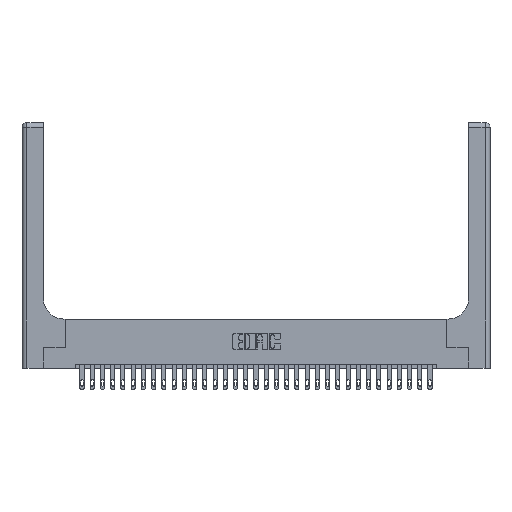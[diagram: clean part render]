
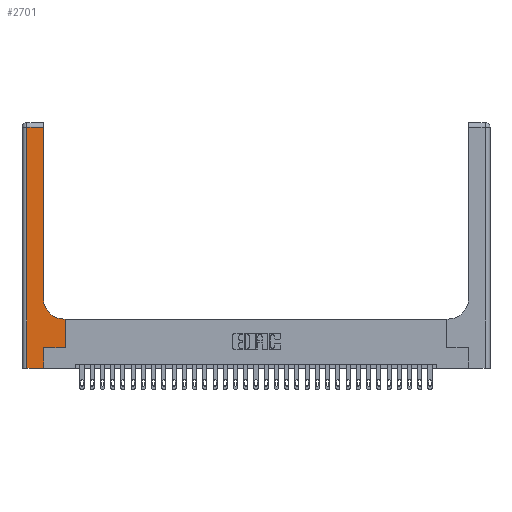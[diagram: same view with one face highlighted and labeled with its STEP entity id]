
A CAD part, top view. The second image highlights one B-rep face of the part: STEP entity #2701.
In plain terms, the highlighted planar face has unit normal (0, 0, 1).
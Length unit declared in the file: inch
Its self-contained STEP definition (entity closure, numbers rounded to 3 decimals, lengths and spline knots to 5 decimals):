
#189 = DIRECTION ( 'NONE',  ( 1., 0., 0. ) ) ;
#437 = LINE ( 'NONE', #23005, #7215 ) ;
#737 = CARTESIAN_POINT ( 'NONE',  ( 0., 0., 0.37 ) ) ;
#1983 = ORIENTED_EDGE ( 'NONE', *, *, #17856, .T. ) ;
#2076 = FACE_OUTER_BOUND ( 'NONE', #5030, .T. ) ;
#2088 = ORIENTED_EDGE ( 'NONE', *, *, #23078, .T. ) ;
#2123 = CARTESIAN_POINT ( 'NONE',  ( 0.265, 0.25, 0.37 ) ) ;
#2350 = CIRCLE ( 'NONE', #26755, 0.25 ) ;
#2701 = ADVANCED_FACE ( 'NONE', ( #2076 ), #20249, .F. ) ;
#3239 = CARTESIAN_POINT ( 'NONE',  ( 0.265, 0., 0.37 ) ) ;
#3316 = DIRECTION ( 'NONE',  ( 0., 0., -1. ) ) ;
#3659 = CARTESIAN_POINT ( 'NONE',  ( 0., 2.94, 0.37 ) ) ;
#3998 = DIRECTION ( 'NONE',  ( 0., 1., 0. ) ) ;
#4167 = VECTOR ( 'NONE', #19620, 39.37008 ) ;
#4446 = DIRECTION ( 'NONE',  ( 0., 0., -1. ) ) ;
#4845 = ORIENTED_EDGE ( 'NONE', *, *, #25050, .T. ) ;
#5030 = EDGE_LOOP ( 'NONE', ( #12765, #10498, #20562, #2088, #4845, #13483, #8958, #1983, #25902 ) ) ;
#5053 = VERTEX_POINT ( 'NONE', #8033 ) ;
#5609 = VECTOR ( 'NONE', #3998, 39.37008 ) ;
#5648 = DIRECTION ( 'NONE',  ( 1., 0., 0. ) ) ;
#6220 = VERTEX_POINT ( 'NONE', #7298 ) ;
#7106 = VECTOR ( 'NONE', #8138, 39.37008 ) ;
#7215 = VECTOR ( 'NONE', #16648, 39.37008 ) ;
#7298 = CARTESIAN_POINT ( 'NONE',  ( 0.528, 0.6, 0.37 ) ) ;
#7432 = CARTESIAN_POINT ( 'NONE',  ( 0.265, 0.25, 0.37 ) ) ;
#8033 = CARTESIAN_POINT ( 'NONE',  ( 0.26, 2.94, 0.37 ) ) ;
#8138 = DIRECTION ( 'NONE',  ( 1., 0., 0. ) ) ;
#8958 = ORIENTED_EDGE ( 'NONE', *, *, #18855, .T. ) ;
#10444 = CARTESIAN_POINT ( 'NONE',  ( 0.51, 0.85, 0.37 ) ) ;
#10498 = ORIENTED_EDGE ( 'NONE', *, *, #15557, .T. ) ;
#10643 = VERTEX_POINT ( 'NONE', #11607 ) ;
#11607 = CARTESIAN_POINT ( 'NONE',  ( 0.06, 2.94, 0.37 ) ) ;
#11711 = VECTOR ( 'NONE', #189, 39.37008 ) ;
#11792 = LINE ( 'NONE', #2123, #11711 ) ;
#12743 = CARTESIAN_POINT ( 'NONE',  ( 0.06, 0., 0.37 ) ) ;
#12765 = ORIENTED_EDGE ( 'NONE', *, *, #24656, .T. ) ;
#13483 = ORIENTED_EDGE ( 'NONE', *, *, #27693, .T. ) ;
#14530 = LINE ( 'NONE', #28483, #4167 ) ;
#15557 = EDGE_CURVE ( 'NONE', #5053, #10643, #23961, .T. ) ;
#15814 = CARTESIAN_POINT ( 'NONE',  ( 0.265, 0., 0.37 ) ) ;
#15904 = VECTOR ( 'NONE', #16498, 39.37008 ) ;
#16498 = DIRECTION ( 'NONE',  ( 0., 1., 0. ) ) ;
#16628 = CARTESIAN_POINT ( 'NONE',  ( 0.26, 0.85, 0.37 ) ) ;
#16648 = DIRECTION ( 'NONE',  ( -1., 0., 0. ) ) ;
#17417 = VECTOR ( 'NONE', #21794, 39.37008 ) ;
#17856 = EDGE_CURVE ( 'NONE', #6220, #26349, #437, .T. ) ;
#18608 = EDGE_CURVE ( 'NONE', #26349, #24909, #2350, .T. ) ;
#18855 = EDGE_CURVE ( 'NONE', #25425, #6220, #23436, .T. ) ;
#18916 = VECTOR ( 'NONE', #24295, 39.37008 ) ;
#19389 = CARTESIAN_POINT ( 'NONE',  ( 0.26, 3., 0.37 ) ) ;
#19423 = EDGE_CURVE ( 'NONE', #10643, #26896, #14530, .T. ) ;
#19620 = DIRECTION ( 'NONE',  ( 0., -1., 0. ) ) ;
#20249 = PLANE ( 'NONE',  #27511 ) ;
#20562 = ORIENTED_EDGE ( 'NONE', *, *, #19423, .T. ) ;
#21213 = CARTESIAN_POINT ( 'NONE',  ( 0.528, 0.25, 0.37 ) ) ;
#21595 = CARTESIAN_POINT ( 'NONE',  ( 0.51, 0.6, 0.37 ) ) ;
#21794 = DIRECTION ( 'NONE',  ( -1., 0., 0. ) ) ;
#23005 = CARTESIAN_POINT ( 'NONE',  ( 0.26, 0.6, 0.37 ) ) ;
#23078 = EDGE_CURVE ( 'NONE', #26896, #27627, #25692, .T. ) ;
#23436 = LINE ( 'NONE', #27933, #15904 ) ;
#23552 = LINE ( 'NONE', #3239, #18916 ) ;
#23961 = LINE ( 'NONE', #3659, #17417 ) ;
#24295 = DIRECTION ( 'NONE',  ( 0., 1., 0. ) ) ;
#24656 = EDGE_CURVE ( 'NONE', #24909, #5053, #26854, .T. ) ;
#24909 = VERTEX_POINT ( 'NONE', #16628 ) ;
#24927 = CARTESIAN_POINT ( 'NONE',  ( 0., 3., 0.37 ) ) ;
#25050 = EDGE_CURVE ( 'NONE', #27627, #26396, #23552, .T. ) ;
#25425 = VERTEX_POINT ( 'NONE', #21213 ) ;
#25692 = LINE ( 'NONE', #737, #7106 ) ;
#25902 = ORIENTED_EDGE ( 'NONE', *, *, #18608, .T. ) ;
#26349 = VERTEX_POINT ( 'NONE', #21595 ) ;
#26396 = VERTEX_POINT ( 'NONE', #7432 ) ;
#26755 = AXIS2_PLACEMENT_3D ( 'NONE', #10444, #3316, #5648 ) ;
#26854 = LINE ( 'NONE', #19389, #5609 ) ;
#26896 = VERTEX_POINT ( 'NONE', #12743 ) ;
#27511 = AXIS2_PLACEMENT_3D ( 'NONE', #24927, #4446, #29263 ) ;
#27627 = VERTEX_POINT ( 'NONE', #15814 ) ;
#27693 = EDGE_CURVE ( 'NONE', #26396, #25425, #11792, .T. ) ;
#27933 = CARTESIAN_POINT ( 'NONE',  ( 0.528, 0.25, 0.37 ) ) ;
#28483 = CARTESIAN_POINT ( 'NONE',  ( 0.06, 3., 0.37 ) ) ;
#29263 = DIRECTION ( 'NONE',  ( -1., 0., 0. ) ) ;
